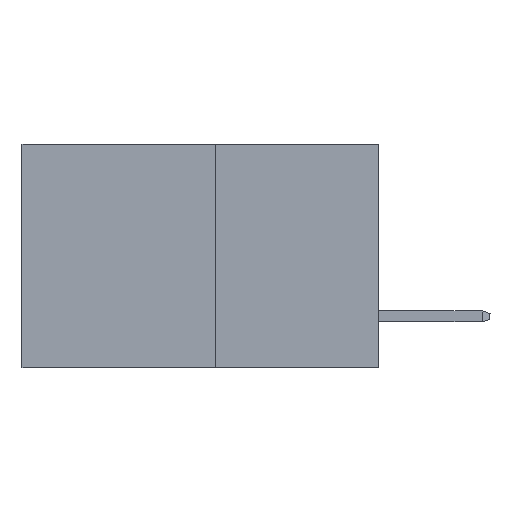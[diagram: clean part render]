
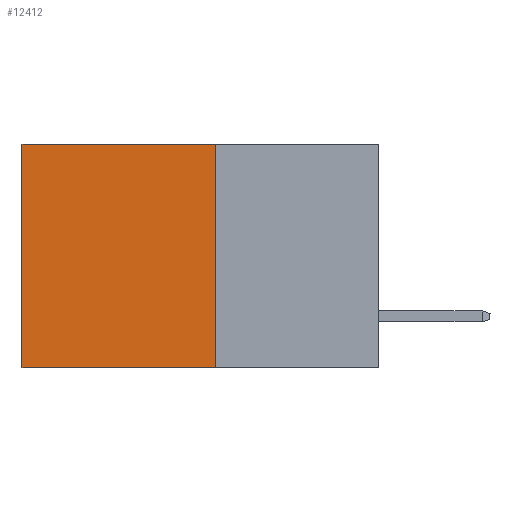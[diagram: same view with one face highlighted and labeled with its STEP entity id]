
A CAD part, left-side view. The second image highlights one B-rep face of the part: STEP entity #12412.
In plain terms, the highlighted planar face has unit normal (-1, 0, 0).
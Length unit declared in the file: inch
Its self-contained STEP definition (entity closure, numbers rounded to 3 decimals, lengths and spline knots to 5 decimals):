
#465 = EDGE_CURVE ( 'NONE', #1783, #4267, #5589, .T. ) ;
#567 = EDGE_CURVE ( 'NONE', #9051, #6355, #8949, .T. ) ;
#878 = VECTOR ( 'NONE', #11182, 39.37008 ) ;
#901 = EDGE_CURVE ( 'NONE', #6355, #4267, #1817, .T. ) ;
#1535 = CARTESIAN_POINT ( 'NONE',  ( 0.277, 0.27, 0. ) ) ;
#1633 = CARTESIAN_POINT ( 'NONE',  ( 0.277, 0.27, -0.37 ) ) ;
#1783 = VERTEX_POINT ( 'NONE', #5098 ) ;
#1817 = LINE ( 'NONE', #8356, #12899 ) ;
#2455 = ORIENTED_EDGE ( 'NONE', *, *, #465, .T. ) ;
#2737 = CARTESIAN_POINT ( 'NONE',  ( 0.277, 0.27, -0.37 ) ) ;
#2782 = DIRECTION ( 'NONE',  ( 1., 0., 0. ) ) ;
#3858 = CARTESIAN_POINT ( 'NONE',  ( 0.277, 0.27, -0.37 ) ) ;
#4267 = VERTEX_POINT ( 'NONE', #6106 ) ;
#5098 = CARTESIAN_POINT ( 'NONE',  ( 0.277, 0.59, 0. ) ) ;
#5589 = LINE ( 'NONE', #8457, #13706 ) ;
#6106 = CARTESIAN_POINT ( 'NONE',  ( 0.277, 0.59, -0.37 ) ) ;
#6128 = VECTOR ( 'NONE', #11599, 39.37008 ) ;
#6355 = VERTEX_POINT ( 'NONE', #3858 ) ;
#8220 = ORIENTED_EDGE ( 'NONE', *, *, #901, .F. ) ;
#8356 = CARTESIAN_POINT ( 'NONE',  ( 0.277, 0.27, -0.37 ) ) ;
#8457 = CARTESIAN_POINT ( 'NONE',  ( 0.277, 0.59, -0.37 ) ) ;
#8554 = ORIENTED_EDGE ( 'NONE', *, *, #11640, .T. ) ;
#8949 = LINE ( 'NONE', #1633, #6128 ) ;
#9051 = VERTEX_POINT ( 'NONE', #13291 ) ;
#9268 = PLANE ( 'NONE',  #9334 ) ;
#9324 = DIRECTION ( 'NONE',  ( 0., 0., -1. ) ) ;
#9334 = AXIS2_PLACEMENT_3D ( 'NONE', #2737, #2782, #10395 ) ;
#10191 = FACE_OUTER_BOUND ( 'NONE', #12295, .T. ) ;
#10395 = DIRECTION ( 'NONE',  ( 0., 0., -1. ) ) ;
#10493 = DIRECTION ( 'NONE',  ( 0., 1., 0. ) ) ;
#11088 = ORIENTED_EDGE ( 'NONE', *, *, #567, .F. ) ;
#11182 = DIRECTION ( 'NONE',  ( 0., 1., 0. ) ) ;
#11599 = DIRECTION ( 'NONE',  ( 0., 0., -1. ) ) ;
#11640 = EDGE_CURVE ( 'NONE', #9051, #1783, #11994, .T. ) ;
#11994 = LINE ( 'NONE', #1535, #878 ) ;
#12295 = EDGE_LOOP ( 'NONE', ( #2455, #8220, #11088, #8554 ) ) ;
#12412 = ADVANCED_FACE ( 'NONE', ( #10191 ), #9268, .F. ) ;
#12899 = VECTOR ( 'NONE', #10493, 39.37008 ) ;
#13291 = CARTESIAN_POINT ( 'NONE',  ( 0.277, 0.27, 0. ) ) ;
#13706 = VECTOR ( 'NONE', #9324, 39.37008 ) ;
